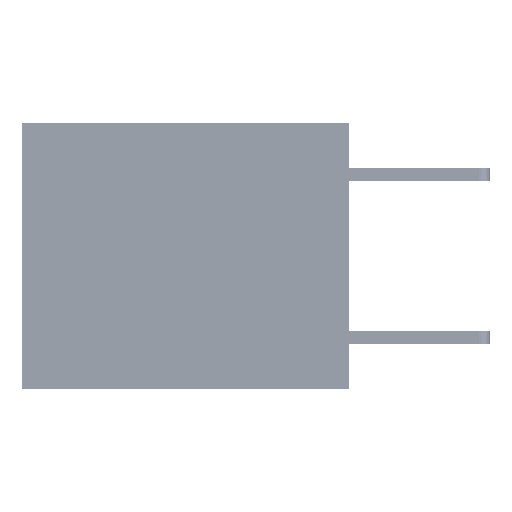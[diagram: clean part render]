
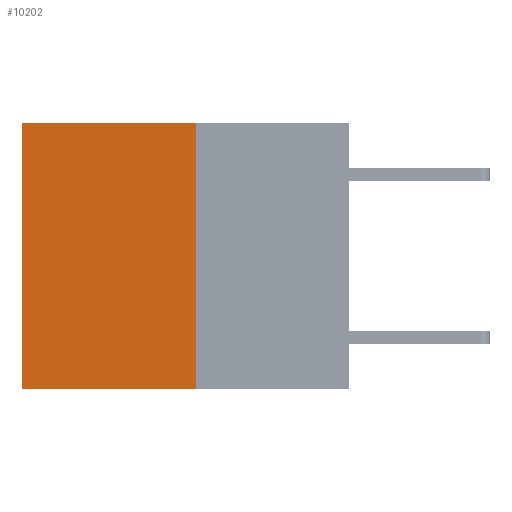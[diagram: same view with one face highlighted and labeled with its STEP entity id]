
A CAD part, left-side view. The second image highlights one B-rep face of the part: STEP entity #10202.
In plain terms, the highlighted planar face has unit normal (-1, 0, 0).
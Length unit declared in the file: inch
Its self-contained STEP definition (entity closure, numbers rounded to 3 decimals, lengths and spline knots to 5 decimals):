
#2068 = CARTESIAN_POINT ( 'NONE',  ( 0.3165, 0.6, 0. ) ) ;
#2531 = CARTESIAN_POINT ( 'NONE',  ( 0.3165, 0.6, -0.49 ) ) ;
#3496 = DIRECTION ( 'NONE',  ( 0., 1., 0. ) ) ;
#4139 = ORIENTED_EDGE ( 'NONE', *, *, #7917, .T. ) ;
#4517 = VECTOR ( 'NONE', #28203, 39.37008 ) ;
#4842 = FACE_OUTER_BOUND ( 'NONE', #6765, .T. ) ;
#6765 = EDGE_LOOP ( 'NONE', ( #4139, #30585, #24825, #23511 ) ) ;
#7917 = EDGE_CURVE ( 'NONE', #19009, #30682, #11955, .T. ) ;
#8408 = VECTOR ( 'NONE', #3496, 39.37008 ) ;
#8789 = PLANE ( 'NONE',  #11767 ) ;
#9124 = CARTESIAN_POINT ( 'NONE',  ( 0.3165, 0.28, -0.49 ) ) ;
#10202 = ADVANCED_FACE ( 'NONE', ( #4842 ), #8789, .F. ) ;
#10475 = CARTESIAN_POINT ( 'NONE',  ( 0.3165, 0.28, -0.49 ) ) ;
#11767 = AXIS2_PLACEMENT_3D ( 'NONE', #34270, #11837, #22745 ) ;
#11837 = DIRECTION ( 'NONE',  ( 1., 0., 0. ) ) ;
#11955 = LINE ( 'NONE', #2531, #4517 ) ;
#12775 = LINE ( 'NONE', #31424, #8408 ) ;
#14629 = CARTESIAN_POINT ( 'NONE',  ( 0.3165, 0.6, -0.49 ) ) ;
#17742 = EDGE_CURVE ( 'NONE', #36076, #19009, #12775, .T. ) ;
#17779 = EDGE_CURVE ( 'NONE', #36076, #31356, #24168, .T. ) ;
#19009 = VERTEX_POINT ( 'NONE', #2068 ) ;
#21252 = DIRECTION ( 'NONE',  ( 0., 0., -1. ) ) ;
#21994 = VECTOR ( 'NONE', #21252, 39.37008 ) ;
#22745 = DIRECTION ( 'NONE',  ( 0., 0., -1. ) ) ;
#23511 = ORIENTED_EDGE ( 'NONE', *, *, #17742, .T. ) ;
#24032 = LINE ( 'NONE', #32683, #32372 ) ;
#24168 = LINE ( 'NONE', #9124, #21994 ) ;
#24825 = ORIENTED_EDGE ( 'NONE', *, *, #17779, .F. ) ;
#27259 = DIRECTION ( 'NONE',  ( 0., 1., 0. ) ) ;
#28203 = DIRECTION ( 'NONE',  ( 0., 0., -1. ) ) ;
#30403 = EDGE_CURVE ( 'NONE', #31356, #30682, #24032, .T. ) ;
#30585 = ORIENTED_EDGE ( 'NONE', *, *, #30403, .F. ) ;
#30682 = VERTEX_POINT ( 'NONE', #14629 ) ;
#31356 = VERTEX_POINT ( 'NONE', #10475 ) ;
#31424 = CARTESIAN_POINT ( 'NONE',  ( 0.3165, 0.28, 0. ) ) ;
#32372 = VECTOR ( 'NONE', #27259, 39.37008 ) ;
#32683 = CARTESIAN_POINT ( 'NONE',  ( 0.3165, 0.28, -0.49 ) ) ;
#34270 = CARTESIAN_POINT ( 'NONE',  ( 0.3165, 0.28, -0.49 ) ) ;
#35447 = CARTESIAN_POINT ( 'NONE',  ( 0.3165, 0.28, 0. ) ) ;
#36076 = VERTEX_POINT ( 'NONE', #35447 ) ;
